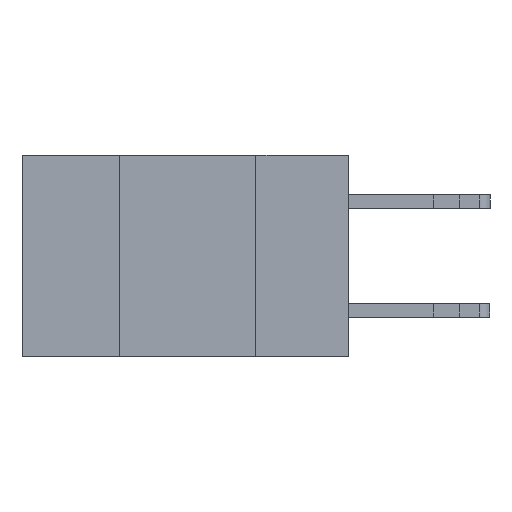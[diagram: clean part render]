
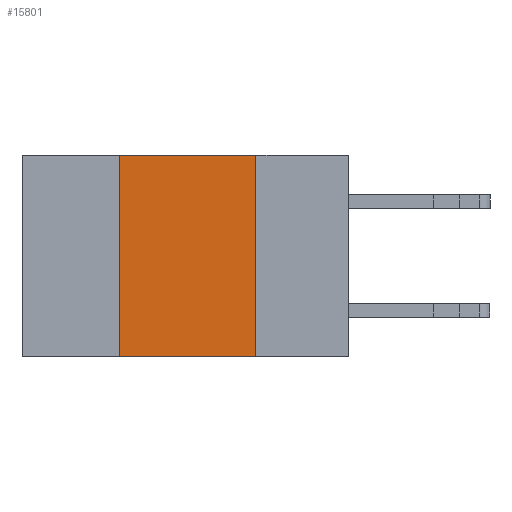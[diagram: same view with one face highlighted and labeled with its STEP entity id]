
A CAD part, left-side view. The second image highlights one B-rep face of the part: STEP entity #15801.
In plain terms, the highlighted planar face has unit normal (-1, 0, 0).
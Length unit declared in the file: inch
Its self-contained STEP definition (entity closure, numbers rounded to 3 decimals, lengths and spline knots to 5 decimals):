
#388 = EDGE_LOOP ( 'NONE', ( #14579, #12297, #16234, #577 ) ) ;
#577 = ORIENTED_EDGE ( 'NONE', *, *, #11375, .T. ) ;
#605 = DIRECTION ( 'NONE',  ( 1., 0., 0. ) ) ;
#1126 = CARTESIAN_POINT ( 'NONE',  ( 0., 0.6, 0. ) ) ;
#1837 = VERTEX_POINT ( 'NONE', #12717 ) ;
#2562 = FACE_OUTER_BOUND ( 'NONE', #388, .T. ) ;
#2940 = EDGE_CURVE ( 'NONE', #11631, #1837, #5898, .T. ) ;
#4544 = DIRECTION ( 'NONE',  ( 0., -1., 0. ) ) ;
#5669 = AXIS2_PLACEMENT_3D ( 'NONE', #10275, #605, #10337 ) ;
#5898 = LINE ( 'NONE', #1126, #12801 ) ;
#6589 = DIRECTION ( 'NONE',  ( 0., 0., 1. ) ) ;
#7019 = VECTOR ( 'NONE', #6589, 39.37008 ) ;
#7685 = VERTEX_POINT ( 'NONE', #10054 ) ;
#8570 = EDGE_CURVE ( 'NONE', #1837, #7685, #14236, .T. ) ;
#8741 = CARTESIAN_POINT ( 'NONE',  ( 0., 0.17, 0. ) ) ;
#8807 = VERTEX_POINT ( 'NONE', #17174 ) ;
#8936 = PLANE ( 'NONE',  #5669 ) ;
#9245 = CARTESIAN_POINT ( 'NONE',  ( 0., 0.42, 0. ) ) ;
#9527 = EDGE_CURVE ( 'NONE', #8807, #11631, #10715, .T. ) ;
#9934 = DIRECTION ( 'NONE',  ( 0., -1., 0. ) ) ;
#10054 = CARTESIAN_POINT ( 'NONE',  ( 0., 0.17, -0.37 ) ) ;
#10275 = CARTESIAN_POINT ( 'NONE',  ( 0., 0.6, 0. ) ) ;
#10337 = DIRECTION ( 'NONE',  ( 0., 0., -1. ) ) ;
#10715 = LINE ( 'NONE', #13430, #7019 ) ;
#11375 = EDGE_CURVE ( 'NONE', #8807, #7685, #13210, .T. ) ;
#11631 = VERTEX_POINT ( 'NONE', #9245 ) ;
#12297 = ORIENTED_EDGE ( 'NONE', *, *, #2940, .F. ) ;
#12717 = CARTESIAN_POINT ( 'NONE',  ( 0., 0.17, 0. ) ) ;
#12801 = VECTOR ( 'NONE', #9934, 39.37008 ) ;
#13210 = LINE ( 'NONE', #14180, #16316 ) ;
#13430 = CARTESIAN_POINT ( 'NONE',  ( 0., 0.42, 0. ) ) ;
#13803 = VECTOR ( 'NONE', #16789, 39.37008 ) ;
#14180 = CARTESIAN_POINT ( 'NONE',  ( 0., 0.6, -0.37 ) ) ;
#14236 = LINE ( 'NONE', #8741, #13803 ) ;
#14579 = ORIENTED_EDGE ( 'NONE', *, *, #8570, .F. ) ;
#15801 = ADVANCED_FACE ( 'NONE', ( #2562 ), #8936, .F. ) ;
#16234 = ORIENTED_EDGE ( 'NONE', *, *, #9527, .F. ) ;
#16316 = VECTOR ( 'NONE', #4544, 39.37008 ) ;
#16789 = DIRECTION ( 'NONE',  ( 0., 0., -1. ) ) ;
#17174 = CARTESIAN_POINT ( 'NONE',  ( 0., 0.42, -0.37 ) ) ;
